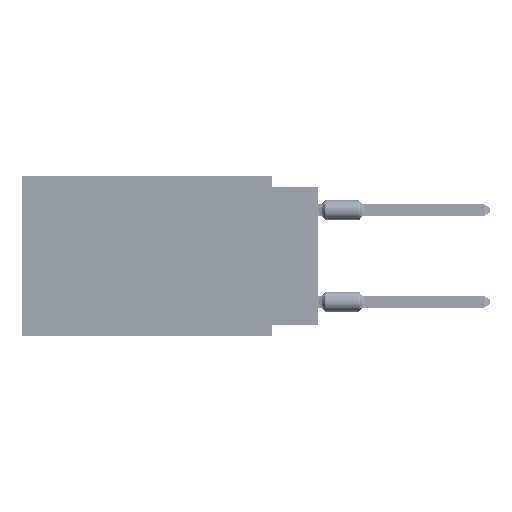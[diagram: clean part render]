
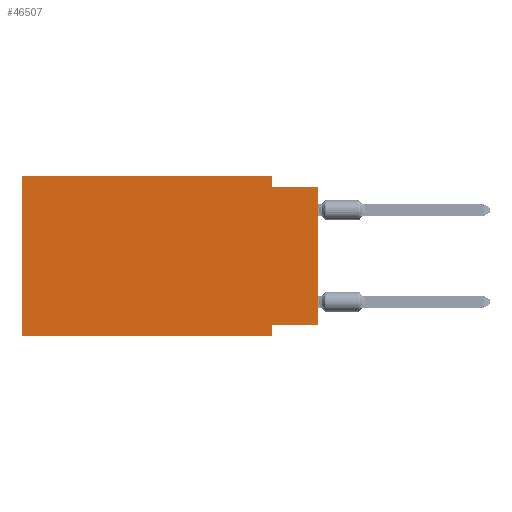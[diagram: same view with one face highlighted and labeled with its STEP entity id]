
A CAD part, left-side view. The second image highlights one B-rep face of the part: STEP entity #46507.
In plain terms, the highlighted planar face has unit normal (-1, 0, 0).
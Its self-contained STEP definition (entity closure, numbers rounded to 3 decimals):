
#557 = EDGE_CURVE ( 'NONE', #12394, #24053, #24248, .T. ) ;
#660 = CARTESIAN_POINT ( 'NONE',  ( 0., 0., -8.255 ) ) ;
#3358 = CARTESIAN_POINT ( 'NONE',  ( 0., 16.383, -8.89 ) ) ;
#5179 = CARTESIAN_POINT ( 'NONE',  ( 0., 2.54, -8.89 ) ) ;
#5216 = FACE_OUTER_BOUND ( 'NONE', #31222, .T. ) ;
#6893 = DIRECTION ( 'NONE',  ( 0., 0., -1. ) ) ;
#7416 = DIRECTION ( 'NONE',  ( 0., -1., 0. ) ) ;
#12394 = VERTEX_POINT ( 'NONE', #3358 ) ;
#12621 = LINE ( 'NONE', #46986, #12784 ) ;
#12784 = VECTOR ( 'NONE', #69729, 1000. ) ;
#15082 = EDGE_CURVE ( 'NONE', #29563, #60417, #12621, .T. ) ;
#15745 = CARTESIAN_POINT ( 'NONE',  ( 0., 0., -0.635 ) ) ;
#15860 = ORIENTED_EDGE ( 'NONE', *, *, #53769, .F. ) ;
#16324 = VECTOR ( 'NONE', #41416, 1000. ) ;
#16992 = VERTEX_POINT ( 'NONE', #69535 ) ;
#18215 = EDGE_CURVE ( 'NONE', #12394, #73041, #48736, .T. ) ;
#19983 = ORIENTED_EDGE ( 'NONE', *, *, #18215, .F. ) ;
#20301 = ORIENTED_EDGE ( 'NONE', *, *, #37081, .F. ) ;
#23743 = DIRECTION ( 'NONE',  ( 0., 0., -1. ) ) ;
#24053 = VERTEX_POINT ( 'NONE', #5179 ) ;
#24248 = LINE ( 'NONE', #29836, #67025 ) ;
#25090 = ORIENTED_EDGE ( 'NONE', *, *, #557, .T. ) ;
#26002 = VECTOR ( 'NONE', #23743, 1000. ) ;
#28733 = PLANE ( 'NONE',  #73088 ) ;
#28860 = VECTOR ( 'NONE', #48997, 1000. ) ;
#29106 = DIRECTION ( 'NONE',  ( 0., 0., -1. ) ) ;
#29563 = VERTEX_POINT ( 'NONE', #660 ) ;
#29836 = CARTESIAN_POINT ( 'NONE',  ( 0., 16.383, -8.89 ) ) ;
#29859 = CARTESIAN_POINT ( 'NONE',  ( 0., 16.383, 0. ) ) ;
#30072 = CARTESIAN_POINT ( 'NONE',  ( 0., 2.54, -8.89 ) ) ;
#30399 = ORIENTED_EDGE ( 'NONE', *, *, #15082, .T. ) ;
#30435 = LINE ( 'NONE', #30072, #26002 ) ;
#31222 = EDGE_LOOP ( 'NONE', ( #30399, #20301, #44637, #62788, #19983, #25090, #65754, #15860 ) ) ;
#31226 = EDGE_CURVE ( 'NONE', #71697, #24053, #30435, .T. ) ;
#32688 = LINE ( 'NONE', #55468, #50082 ) ;
#36746 = CARTESIAN_POINT ( 'NONE',  ( 0., 0., -8.255 ) ) ;
#37081 = EDGE_CURVE ( 'NONE', #16992, #60417, #49363, .T. ) ;
#40608 = VECTOR ( 'NONE', #71440, 1000. ) ;
#41416 = DIRECTION ( 'NONE',  ( 0., -1., 0. ) ) ;
#42725 = VECTOR ( 'NONE', #43113, 1000. ) ;
#43113 = DIRECTION ( 'NONE',  ( 0., 0., 1. ) ) ;
#44637 = ORIENTED_EDGE ( 'NONE', *, *, #53603, .F. ) ;
#46507 = ADVANCED_FACE ( 'NONE', ( #5216 ), #28733, .F. ) ;
#46986 = CARTESIAN_POINT ( 'NONE',  ( 0., 0., 0. ) ) ;
#48736 = LINE ( 'NONE', #66973, #42725 ) ;
#48997 = DIRECTION ( 'NONE',  ( 0., -1., 0. ) ) ;
#49363 = LINE ( 'NONE', #15745, #28860 ) ;
#50082 = VECTOR ( 'NONE', #6893, 1000. ) ;
#50756 = VERTEX_POINT ( 'NONE', #51347 ) ;
#50764 = DIRECTION ( 'NONE',  ( 1., 0., 0. ) ) ;
#50977 = CARTESIAN_POINT ( 'NONE',  ( 0., 0., -0.635 ) ) ;
#51347 = CARTESIAN_POINT ( 'NONE',  ( 0., 2.54, 0. ) ) ;
#52933 = EDGE_CURVE ( 'NONE', #73041, #50756, #69051, .T. ) ;
#53603 = EDGE_CURVE ( 'NONE', #50756, #16992, #32688, .T. ) ;
#53769 = EDGE_CURVE ( 'NONE', #29563, #71697, #65845, .T. ) ;
#55468 = CARTESIAN_POINT ( 'NONE',  ( 0., 2.54, 0. ) ) ;
#60417 = VERTEX_POINT ( 'NONE', #50977 ) ;
#62788 = ORIENTED_EDGE ( 'NONE', *, *, #52933, .F. ) ;
#65754 = ORIENTED_EDGE ( 'NONE', *, *, #31226, .F. ) ;
#65845 = LINE ( 'NONE', #36746, #40608 ) ;
#66973 = CARTESIAN_POINT ( 'NONE',  ( 0., 16.383, 0. ) ) ;
#67025 = VECTOR ( 'NONE', #7416, 1000. ) ;
#69033 = CARTESIAN_POINT ( 'NONE',  ( 0., 16.383, 0. ) ) ;
#69051 = LINE ( 'NONE', #29859, #16324 ) ;
#69535 = CARTESIAN_POINT ( 'NONE',  ( 0., 2.54, -0.635 ) ) ;
#69729 = DIRECTION ( 'NONE',  ( 0., 0., 1. ) ) ;
#70890 = CARTESIAN_POINT ( 'NONE',  ( 0., 2.54, -8.255 ) ) ;
#71440 = DIRECTION ( 'NONE',  ( 0., 1., 0. ) ) ;
#71697 = VERTEX_POINT ( 'NONE', #70890 ) ;
#71756 = CARTESIAN_POINT ( 'NONE',  ( 0., 16.383, 0. ) ) ;
#73041 = VERTEX_POINT ( 'NONE', #71756 ) ;
#73088 = AXIS2_PLACEMENT_3D ( 'NONE', #69033, #50764, #29106 ) ;
